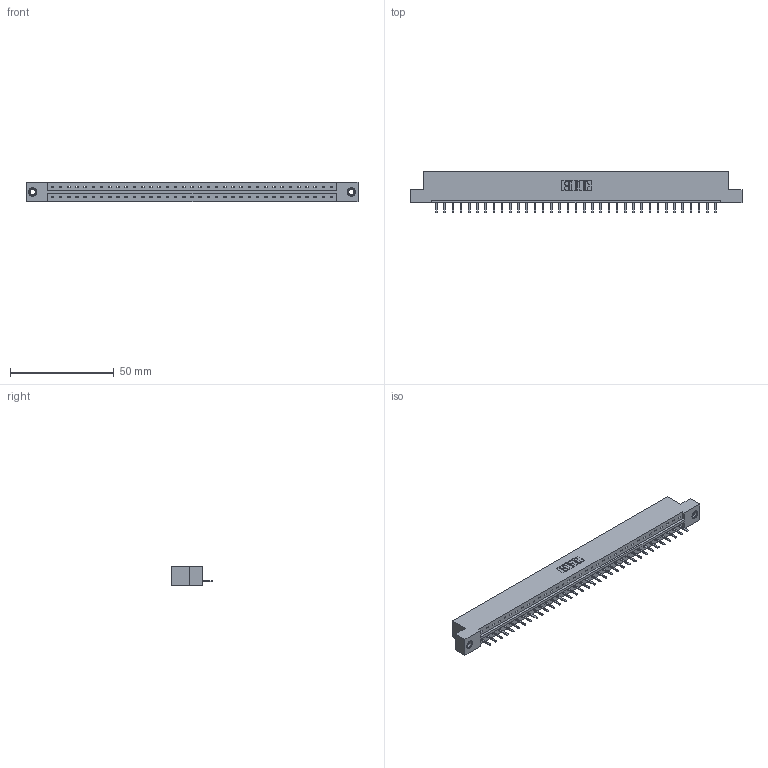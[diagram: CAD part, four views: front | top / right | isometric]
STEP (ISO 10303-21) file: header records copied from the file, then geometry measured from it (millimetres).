
FILE_DESCRIPTION (( 'STEP AP203' ), '1' );
FILE_NAME ('333-035-520-107.STEP', '2018-08-02T23:19:26', ( '' ), ( '' ), 'SwSTEP 2.0', 'SolidWorks 2016', '' );
FILE_SCHEMA (( 'CONFIG_CONTROL_DESIGN' ));
Length unit declared in the file: inch
Products named in the file (4): 333-035-520-107; 333 Part_Flush - .156 Dia - TI; 345-292-001_345-293-120; 345-250-001_345-250-005-103
Assembly tree (38 placements, depth 2):
  333-035-520-107
    333 Part_Flush - .156 Dia - TI
    345-292-001_345-293-120  x35
    345-250-001_345-250-005-103  x2
Bounding box: 160.22 x 20.02 x 9.4 mm (x, y, z)
Volume: 15948.6 mm3; surface area: 16894.6 mm2
Topology: 38 solids, 38 shells, 2344 faces, 6887 edges, 4490 vertices
Faces by surface type: plane 1642, cylinder 686, cone 12, torus 4
Entity records: 23602 total; most frequent: CARTESIAN_POINT 4066, ORIENTED_EDGE 4018, DIRECTION 3465, EDGE_CURVE 2009, LINE 1857, VECTOR 1857, VERTEX_POINT 1332, AXIS2_PLACEMENT_3D 804
